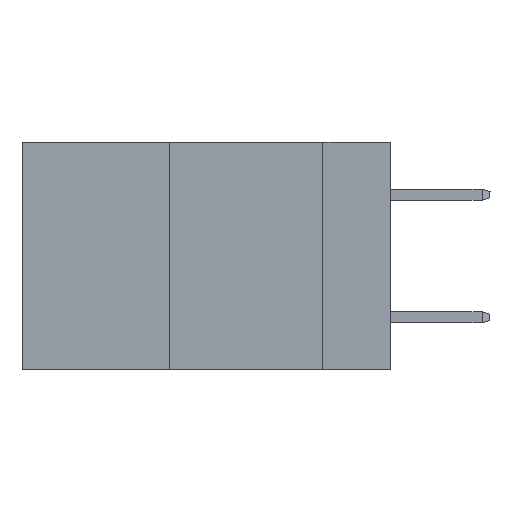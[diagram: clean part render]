
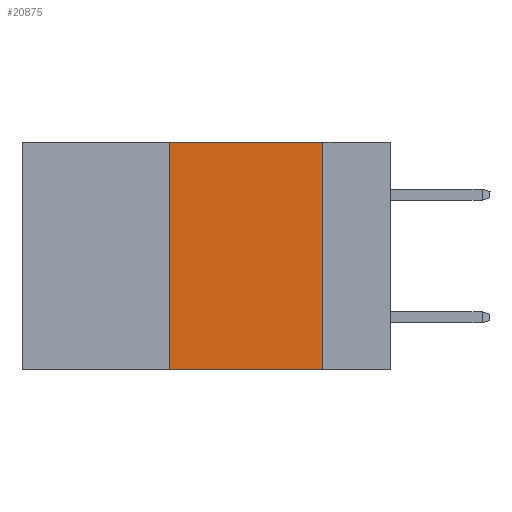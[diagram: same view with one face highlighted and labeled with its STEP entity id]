
A CAD part, left-side view. The second image highlights one B-rep face of the part: STEP entity #20875.
In plain terms, the highlighted planar face has unit normal (-1, 0, 0).
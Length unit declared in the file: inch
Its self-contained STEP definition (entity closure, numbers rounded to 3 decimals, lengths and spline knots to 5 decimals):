
#1466 = PLANE ( 'NONE',  #23200 ) ;
#2313 = EDGE_LOOP ( 'NONE', ( #15316, #22659, #22075, #19605 ) ) ;
#2920 = LINE ( 'NONE', #10756, #23962 ) ;
#3432 = FACE_OUTER_BOUND ( 'NONE', #2313, .T. ) ;
#4740 = EDGE_CURVE ( 'NONE', #20776, #10126, #2920, .T. ) ;
#5494 = CARTESIAN_POINT ( 'NONE',  ( 0., 0.36, 0. ) ) ;
#5555 = VERTEX_POINT ( 'NONE', #16673 ) ;
#5927 = VERTEX_POINT ( 'NONE', #8420 ) ;
#6305 = LINE ( 'NONE', #8662, #20716 ) ;
#7078 = VECTOR ( 'NONE', #7596, 39.37008 ) ;
#7087 = CARTESIAN_POINT ( 'NONE',  ( 0., 0.36, 0. ) ) ;
#7207 = LINE ( 'NONE', #17251, #7078 ) ;
#7596 = DIRECTION ( 'NONE',  ( 0., 0., -1. ) ) ;
#7782 = EDGE_CURVE ( 'NONE', #5927, #5555, #6305, .T. ) ;
#8420 = CARTESIAN_POINT ( 'NONE',  ( 0., 0.36, -0.37 ) ) ;
#8662 = CARTESIAN_POINT ( 'NONE',  ( 0., 0.6, -0.37 ) ) ;
#9423 = CARTESIAN_POINT ( 'NONE',  ( 0., 0.6, 0. ) ) ;
#10126 = VERTEX_POINT ( 'NONE', #25041 ) ;
#10756 = CARTESIAN_POINT ( 'NONE',  ( 0., 0.6, 0. ) ) ;
#12444 = DIRECTION ( 'NONE',  ( 0., -1., 0. ) ) ;
#15103 = VECTOR ( 'NONE', #19601, 39.37008 ) ;
#15316 = ORIENTED_EDGE ( 'NONE', *, *, #24876, .F. ) ;
#15813 = EDGE_CURVE ( 'NONE', #5927, #20776, #17503, .T. ) ;
#16673 = CARTESIAN_POINT ( 'NONE',  ( 0., 0.11, -0.37 ) ) ;
#17251 = CARTESIAN_POINT ( 'NONE',  ( 0., 0.11, 0. ) ) ;
#17503 = LINE ( 'NONE', #5494, #15103 ) ;
#18984 = DIRECTION ( 'NONE',  ( 0., -1., 0. ) ) ;
#19601 = DIRECTION ( 'NONE',  ( 0., 0., 1. ) ) ;
#19605 = ORIENTED_EDGE ( 'NONE', *, *, #7782, .T. ) ;
#20716 = VECTOR ( 'NONE', #12444, 39.37008 ) ;
#20776 = VERTEX_POINT ( 'NONE', #7087 ) ;
#20875 = ADVANCED_FACE ( 'NONE', ( #3432 ), #1466, .F. ) ;
#22075 = ORIENTED_EDGE ( 'NONE', *, *, #15813, .F. ) ;
#22659 = ORIENTED_EDGE ( 'NONE', *, *, #4740, .F. ) ;
#23200 = AXIS2_PLACEMENT_3D ( 'NONE', #9423, #25615, #25737 ) ;
#23962 = VECTOR ( 'NONE', #18984, 39.37008 ) ;
#24876 = EDGE_CURVE ( 'NONE', #10126, #5555, #7207, .T. ) ;
#25041 = CARTESIAN_POINT ( 'NONE',  ( 0., 0.11, 0. ) ) ;
#25615 = DIRECTION ( 'NONE',  ( 1., 0., 0. ) ) ;
#25737 = DIRECTION ( 'NONE',  ( 0., 0., -1. ) ) ;
